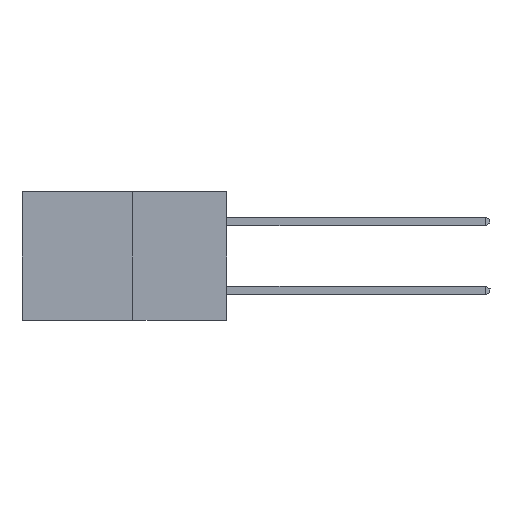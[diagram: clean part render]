
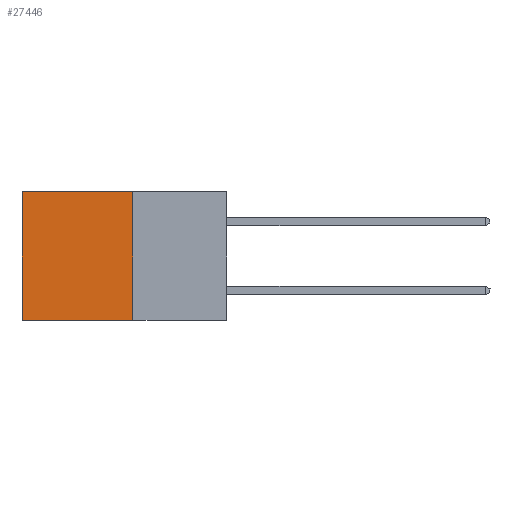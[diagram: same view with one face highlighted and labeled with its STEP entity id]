
A CAD part, left-side view. The second image highlights one B-rep face of the part: STEP entity #27446.
In plain terms, the highlighted planar face has unit normal (-1, 0, 0).
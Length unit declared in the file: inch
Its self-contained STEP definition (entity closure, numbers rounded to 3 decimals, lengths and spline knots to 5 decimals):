
#870 = VERTEX_POINT ( 'NONE', #13504 ) ;
#922 = DIRECTION ( 'NONE',  ( 0., 0., -1. ) ) ;
#1495 = FACE_OUTER_BOUND ( 'NONE', #7956, .T. ) ;
#1557 = VECTOR ( 'NONE', #6879, 39.37008 ) ;
#3598 = VECTOR ( 'NONE', #14783, 39.37008 ) ;
#6136 = CARTESIAN_POINT ( 'NONE',  ( 0.277, 0.27, 0. ) ) ;
#6879 = DIRECTION ( 'NONE',  ( 0., 0., -1. ) ) ;
#7359 = LINE ( 'NONE', #13292, #1557 ) ;
#7507 = EDGE_CURVE ( 'NONE', #25531, #870, #7359, .T. ) ;
#7956 = EDGE_LOOP ( 'NONE', ( #25689, #19335, #13553, #11866 ) ) ;
#8456 = CARTESIAN_POINT ( 'NONE',  ( 0.277, 0.59, 0. ) ) ;
#8621 = CARTESIAN_POINT ( 'NONE',  ( 0.277, 0.27, -0.37 ) ) ;
#10742 = DIRECTION ( 'NONE',  ( 0., 1., 0. ) ) ;
#10805 = DIRECTION ( 'NONE',  ( 1., 0., 0. ) ) ;
#11866 = ORIENTED_EDGE ( 'NONE', *, *, #17948, .T. ) ;
#12620 = VERTEX_POINT ( 'NONE', #27598 ) ;
#12810 = VECTOR ( 'NONE', #10742, 39.37008 ) ;
#13292 = CARTESIAN_POINT ( 'NONE',  ( 0.277, 0.27, -0.37 ) ) ;
#13471 = LINE ( 'NONE', #17043, #12810 ) ;
#13504 = CARTESIAN_POINT ( 'NONE',  ( 0.277, 0.27, -0.37 ) ) ;
#13553 = ORIENTED_EDGE ( 'NONE', *, *, #7507, .F. ) ;
#13879 = CARTESIAN_POINT ( 'NONE',  ( 0.277, 0.59, -0.37 ) ) ;
#13925 = VERTEX_POINT ( 'NONE', #8456 ) ;
#14783 = DIRECTION ( 'NONE',  ( 0., 1., 0. ) ) ;
#17043 = CARTESIAN_POINT ( 'NONE',  ( 0.277, 0.27, -0.37 ) ) ;
#17054 = EDGE_CURVE ( 'NONE', #13925, #12620, #21453, .T. ) ;
#17948 = EDGE_CURVE ( 'NONE', #25531, #13925, #20708, .T. ) ;
#19335 = ORIENTED_EDGE ( 'NONE', *, *, #24758, .F. ) ;
#20708 = LINE ( 'NONE', #6136, #3598 ) ;
#20768 = VECTOR ( 'NONE', #922, 39.37008 ) ;
#21407 = PLANE ( 'NONE',  #27567 ) ;
#21453 = LINE ( 'NONE', #13879, #20768 ) ;
#24758 = EDGE_CURVE ( 'NONE', #870, #12620, #13471, .T. ) ;
#25531 = VERTEX_POINT ( 'NONE', #25764 ) ;
#25685 = DIRECTION ( 'NONE',  ( 0., 0., -1. ) ) ;
#25689 = ORIENTED_EDGE ( 'NONE', *, *, #17054, .T. ) ;
#25764 = CARTESIAN_POINT ( 'NONE',  ( 0.277, 0.27, 0. ) ) ;
#27446 = ADVANCED_FACE ( 'NONE', ( #1495 ), #21407, .F. ) ;
#27567 = AXIS2_PLACEMENT_3D ( 'NONE', #8621, #10805, #25685 ) ;
#27598 = CARTESIAN_POINT ( 'NONE',  ( 0.277, 0.59, -0.37 ) ) ;
